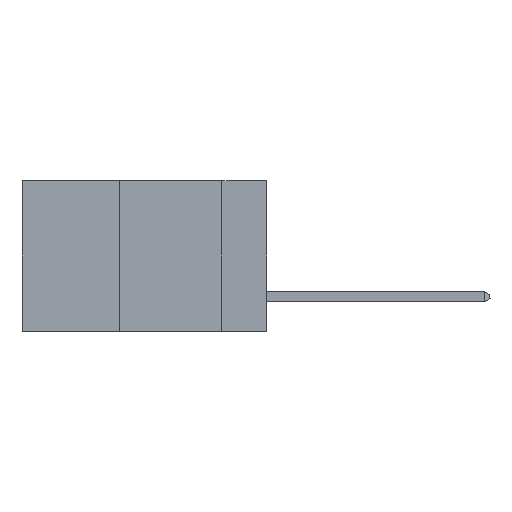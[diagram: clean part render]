
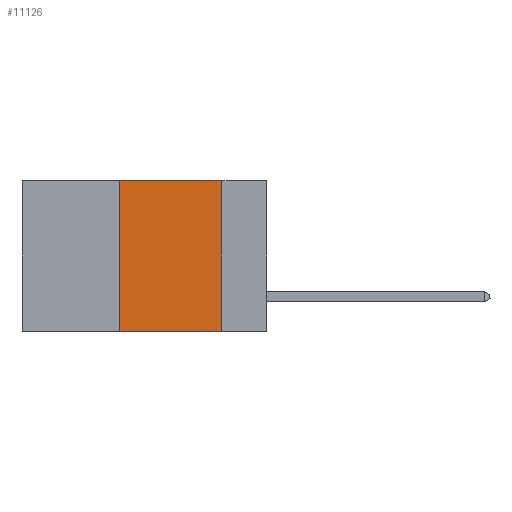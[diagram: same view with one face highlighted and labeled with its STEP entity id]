
A CAD part, left-side view. The second image highlights one B-rep face of the part: STEP entity #11126.
In plain terms, the highlighted planar face has unit normal (-1, 0, 0).
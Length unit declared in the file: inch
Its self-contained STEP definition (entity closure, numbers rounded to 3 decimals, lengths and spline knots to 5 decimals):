
#433 = ORIENTED_EDGE ( 'NONE', *, *, #11749, .T. ) ;
#1769 = VECTOR ( 'NONE', #16986, 39.37008 ) ;
#1821 = DIRECTION ( 'NONE',  ( 0., 0., -1. ) ) ;
#3520 = CARTESIAN_POINT ( 'NONE',  ( 0., 0.6, -0.37 ) ) ;
#3737 = EDGE_CURVE ( 'NONE', #20010, #14172, #9455, .T. ) ;
#4234 = CARTESIAN_POINT ( 'NONE',  ( 0., 0.36, 0. ) ) ;
#4455 = CARTESIAN_POINT ( 'NONE',  ( 0., 0.36, 0. ) ) ;
#5133 = VERTEX_POINT ( 'NONE', #9672 ) ;
#6093 = DIRECTION ( 'NONE',  ( 0., -1., 0. ) ) ;
#7337 = EDGE_CURVE ( 'NONE', #14172, #22147, #13908, .T. ) ;
#7502 = LINE ( 'NONE', #3520, #1769 ) ;
#7794 = ORIENTED_EDGE ( 'NONE', *, *, #7337, .F. ) ;
#9455 = LINE ( 'NONE', #4234, #10270 ) ;
#9672 = CARTESIAN_POINT ( 'NONE',  ( 0., 0.11, -0.37 ) ) ;
#10270 = VECTOR ( 'NONE', #19910, 39.37008 ) ;
#11126 = ADVANCED_FACE ( 'NONE', ( #15366 ), #17914, .F. ) ;
#11211 = DIRECTION ( 'NONE',  ( 1., 0., 0. ) ) ;
#11234 = CARTESIAN_POINT ( 'NONE',  ( 0., 0.6, 0. ) ) ;
#11387 = ORIENTED_EDGE ( 'NONE', *, *, #18884, .F. ) ;
#11749 = EDGE_CURVE ( 'NONE', #20010, #5133, #7502, .T. ) ;
#12851 = EDGE_LOOP ( 'NONE', ( #11387, #7794, #14319, #433 ) ) ;
#13908 = LINE ( 'NONE', #11234, #21207 ) ;
#14172 = VERTEX_POINT ( 'NONE', #4455 ) ;
#14319 = ORIENTED_EDGE ( 'NONE', *, *, #3737, .F. ) ;
#14992 = CARTESIAN_POINT ( 'NONE',  ( 0., 0.11, 0. ) ) ;
#15366 = FACE_OUTER_BOUND ( 'NONE', #12851, .T. ) ;
#16986 = DIRECTION ( 'NONE',  ( 0., -1., 0. ) ) ;
#16997 = LINE ( 'NONE', #19158, #20509 ) ;
#17914 = PLANE ( 'NONE',  #19944 ) ;
#18143 = DIRECTION ( 'NONE',  ( 0., 0., -1. ) ) ;
#18884 = EDGE_CURVE ( 'NONE', #22147, #5133, #16997, .T. ) ;
#19158 = CARTESIAN_POINT ( 'NONE',  ( 0., 0.11, 0. ) ) ;
#19910 = DIRECTION ( 'NONE',  ( 0., 0., 1. ) ) ;
#19944 = AXIS2_PLACEMENT_3D ( 'NONE', #21536, #11211, #18143 ) ;
#20010 = VERTEX_POINT ( 'NONE', #22397 ) ;
#20509 = VECTOR ( 'NONE', #1821, 39.37008 ) ;
#21207 = VECTOR ( 'NONE', #6093, 39.37008 ) ;
#21536 = CARTESIAN_POINT ( 'NONE',  ( 0., 0.6, 0. ) ) ;
#22147 = VERTEX_POINT ( 'NONE', #14992 ) ;
#22397 = CARTESIAN_POINT ( 'NONE',  ( 0., 0.36, -0.37 ) ) ;
